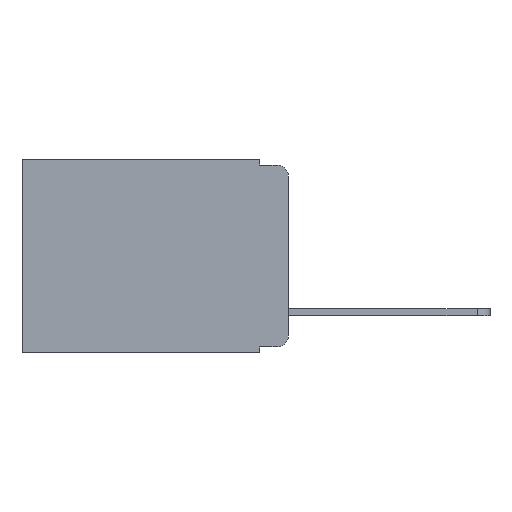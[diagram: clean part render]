
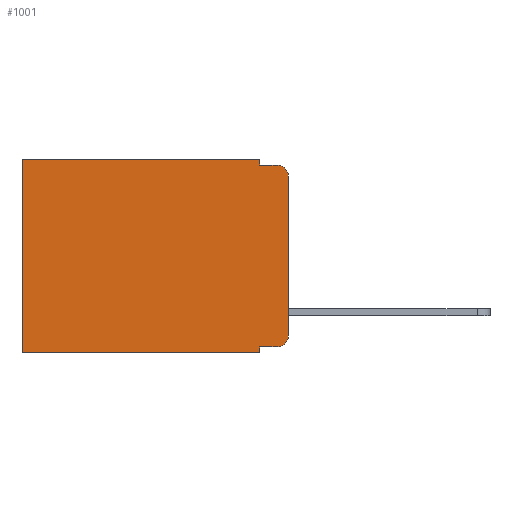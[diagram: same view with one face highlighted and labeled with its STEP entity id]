
A CAD part, left-side view. The second image highlights one B-rep face of the part: STEP entity #1001.
In plain terms, the highlighted planar face has unit normal (-1, 0, 0).
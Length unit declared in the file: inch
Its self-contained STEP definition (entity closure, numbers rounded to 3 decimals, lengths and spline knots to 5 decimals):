
#131 = ORIENTED_EDGE ( 'NONE', *, *, #226, .T. ) ;
#186 = ORIENTED_EDGE ( 'NONE', *, *, #13477, .F. ) ;
#191 = LINE ( 'NONE', #2486, #10463 ) ;
#226 = EDGE_CURVE ( 'NONE', #14588, #11380, #6420, .T. ) ;
#305 = LINE ( 'NONE', #16947, #7492 ) ;
#348 = LINE ( 'NONE', #8833, #14084 ) ;
#682 = CARTESIAN_POINT ( 'NONE',  ( 0.298, 0., 0. ) ) ;
#729 = DIRECTION ( 'NONE',  ( -1., 0., 0. ) ) ;
#749 = DIRECTION ( 'NONE',  ( 0., -1., 0. ) ) ;
#1001 = ADVANCED_FACE ( 'NONE', ( #1744 ), #4799, .F. ) ;
#1097 = EDGE_CURVE ( 'NONE', #11578, #1776, #6806, .T. ) ;
#1122 = DIRECTION ( 'NONE',  ( 0., 0., -1. ) ) ;
#1595 = ORIENTED_EDGE ( 'NONE', *, *, #1097, .F. ) ;
#1744 = FACE_OUTER_BOUND ( 'NONE', #4710, .T. ) ;
#1776 = VERTEX_POINT ( 'NONE', #16129 ) ;
#2168 = CARTESIAN_POINT ( 'NONE',  ( 0.298, 0.473, -0.343 ) ) ;
#2298 = CIRCLE ( 'NONE', #11116, 0.02 ) ;
#2486 = CARTESIAN_POINT ( 'NONE',  ( 0.298, 0., -0.343 ) ) ;
#2614 = VERTEX_POINT ( 'NONE', #11674 ) ;
#2903 = DIRECTION ( 'NONE',  ( -1., 0., 0. ) ) ;
#2904 = EDGE_CURVE ( 'NONE', #15454, #1776, #2298, .T. ) ;
#3252 = AXIS2_PLACEMENT_3D ( 'NONE', #682, #4818, #12903 ) ;
#3329 = LINE ( 'NONE', #3356, #6935 ) ;
#3356 = CARTESIAN_POINT ( 'NONE',  ( 0.298, 0.473, 0. ) ) ;
#3834 = DIRECTION ( 'NONE',  ( 0., 1., 0. ) ) ;
#3888 = ORIENTED_EDGE ( 'NONE', *, *, #7767, .T. ) ;
#4062 = ORIENTED_EDGE ( 'NONE', *, *, #2904, .T. ) ;
#4420 = ORIENTED_EDGE ( 'NONE', *, *, #9559, .T. ) ;
#4661 = CARTESIAN_POINT ( 'NONE',  ( 0.298, 0., 0. ) ) ;
#4710 = EDGE_LOOP ( 'NONE', ( #6195, #4062, #1595, #8774, #131, #9407, #186, #15949, #4420, #3888 ) ) ;
#4718 = DIRECTION ( 'NONE',  ( 0., 0., -1. ) ) ;
#4799 = PLANE ( 'NONE',  #3252 ) ;
#4818 = DIRECTION ( 'NONE',  ( 1., 0., 0. ) ) ;
#5545 = DIRECTION ( 'NONE',  ( 0., 0., -1. ) ) ;
#5838 = CARTESIAN_POINT ( 'NONE',  ( 0.298, 0.02, -0.333 ) ) ;
#5898 = VECTOR ( 'NONE', #10178, 39.37008 ) ;
#5980 = CARTESIAN_POINT ( 'NONE',  ( 0.298, 0., -0.313 ) ) ;
#6195 = ORIENTED_EDGE ( 'NONE', *, *, #8314, .F. ) ;
#6420 = LINE ( 'NONE', #4661, #16023 ) ;
#6806 = LINE ( 'NONE', #10464, #13375 ) ;
#6860 = VERTEX_POINT ( 'NONE', #2168 ) ;
#6935 = VECTOR ( 'NONE', #4718, 39.37008 ) ;
#7492 = VECTOR ( 'NONE', #1122, 39.37008 ) ;
#7767 = EDGE_CURVE ( 'NONE', #9431, #15633, #11922, .T. ) ;
#8307 = CARTESIAN_POINT ( 'NONE',  ( 0.298, 0.051, -0.333 ) ) ;
#8314 = EDGE_CURVE ( 'NONE', #15454, #15633, #13316, .T. ) ;
#8464 = LINE ( 'NONE', #13450, #11964 ) ;
#8716 = VERTEX_POINT ( 'NONE', #8307 ) ;
#8774 = ORIENTED_EDGE ( 'NONE', *, *, #16480, .F. ) ;
#8816 = CARTESIAN_POINT ( 'NONE',  ( 0.298, 0.02, -0.03 ) ) ;
#8833 = CARTESIAN_POINT ( 'NONE',  ( 0.298, 0.051, -0.333 ) ) ;
#9320 = CARTESIAN_POINT ( 'NONE',  ( 0.298, 0.051, -0.01 ) ) ;
#9407 = ORIENTED_EDGE ( 'NONE', *, *, #13905, .T. ) ;
#9431 = VERTEX_POINT ( 'NONE', #5838 ) ;
#9492 = CARTESIAN_POINT ( 'NONE',  ( 0.298, 0., -0.03 ) ) ;
#9559 = EDGE_CURVE ( 'NONE', #8716, #9431, #348, .T. ) ;
#10128 = DIRECTION ( 'NONE',  ( 0., 0., -1. ) ) ;
#10178 = DIRECTION ( 'NONE',  ( 0., 0., -1. ) ) ;
#10463 = VECTOR ( 'NONE', #3834, 39.37008 ) ;
#10464 = CARTESIAN_POINT ( 'NONE',  ( 0.298, 0.051, -0.01 ) ) ;
#10920 = CARTESIAN_POINT ( 'NONE',  ( 0.298, 0.02, -0.313 ) ) ;
#11116 = AXIS2_PLACEMENT_3D ( 'NONE', #8816, #729, #10128 ) ;
#11380 = VERTEX_POINT ( 'NONE', #16618 ) ;
#11507 = CARTESIAN_POINT ( 'NONE',  ( 0.298, 0., 0. ) ) ;
#11578 = VERTEX_POINT ( 'NONE', #9320 ) ;
#11674 = CARTESIAN_POINT ( 'NONE',  ( 0.298, 0.051, -0.343 ) ) ;
#11922 = CIRCLE ( 'NONE', #13492, 0.02 ) ;
#11964 = VECTOR ( 'NONE', #5545, 39.37008 ) ;
#12176 = EDGE_CURVE ( 'NONE', #8716, #2614, #8464, .T. ) ;
#12227 = DIRECTION ( 'NONE',  ( 0., 0., -1. ) ) ;
#12797 = CARTESIAN_POINT ( 'NONE',  ( 0.298, 0.051, 0. ) ) ;
#12903 = DIRECTION ( 'NONE',  ( 0., 0., -1. ) ) ;
#13316 = LINE ( 'NONE', #11507, #5898 ) ;
#13375 = VECTOR ( 'NONE', #13821, 39.37008 ) ;
#13450 = CARTESIAN_POINT ( 'NONE',  ( 0.298, 0.051, 0. ) ) ;
#13477 = EDGE_CURVE ( 'NONE', #2614, #6860, #191, .T. ) ;
#13492 = AXIS2_PLACEMENT_3D ( 'NONE', #10920, #2903, #12227 ) ;
#13821 = DIRECTION ( 'NONE',  ( 0., -1., 0. ) ) ;
#13905 = EDGE_CURVE ( 'NONE', #11380, #6860, #3329, .T. ) ;
#14032 = DIRECTION ( 'NONE',  ( 0., 1., 0. ) ) ;
#14084 = VECTOR ( 'NONE', #749, 39.37008 ) ;
#14588 = VERTEX_POINT ( 'NONE', #12797 ) ;
#15454 = VERTEX_POINT ( 'NONE', #9492 ) ;
#15633 = VERTEX_POINT ( 'NONE', #5980 ) ;
#15949 = ORIENTED_EDGE ( 'NONE', *, *, #12176, .F. ) ;
#16023 = VECTOR ( 'NONE', #14032, 39.37008 ) ;
#16129 = CARTESIAN_POINT ( 'NONE',  ( 0.298, 0.02, -0.01 ) ) ;
#16480 = EDGE_CURVE ( 'NONE', #14588, #11578, #305, .T. ) ;
#16618 = CARTESIAN_POINT ( 'NONE',  ( 0.298, 0.473, 0. ) ) ;
#16947 = CARTESIAN_POINT ( 'NONE',  ( 0.298, 0.051, 0. ) ) ;
